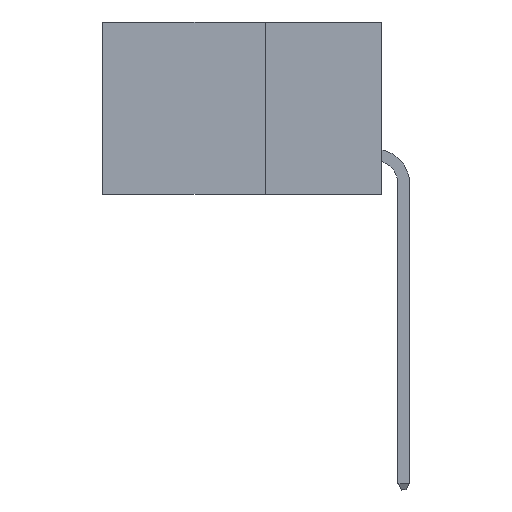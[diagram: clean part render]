
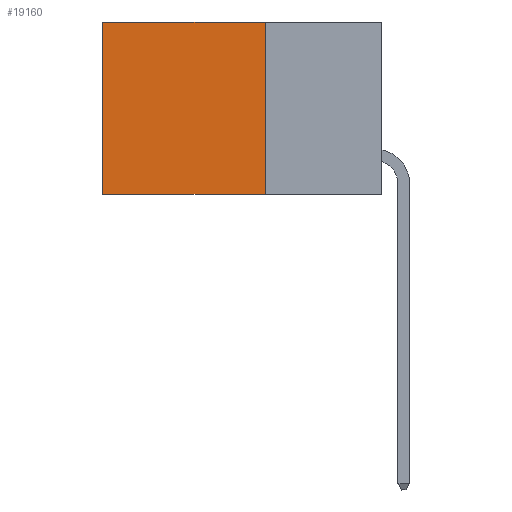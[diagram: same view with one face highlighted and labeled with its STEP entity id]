
A CAD part, left-side view. The second image highlights one B-rep face of the part: STEP entity #19160.
In plain terms, the highlighted planar face has unit normal (-1, 0, 0).
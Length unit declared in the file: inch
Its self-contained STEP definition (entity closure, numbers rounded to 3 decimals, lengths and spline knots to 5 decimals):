
#1195 = DIRECTION ( 'NONE',  ( 0., 0., -1. ) ) ;
#1958 = DIRECTION ( 'NONE',  ( 1., 0., 0. ) ) ;
#2060 = LINE ( 'NONE', #19377, #6332 ) ;
#2730 = ORIENTED_EDGE ( 'NONE', *, *, #21074, .F. ) ;
#3706 = CARTESIAN_POINT ( 'NONE',  ( 0.2875, 0.6, -0.37 ) ) ;
#4814 = VERTEX_POINT ( 'NONE', #15889 ) ;
#6022 = VERTEX_POINT ( 'NONE', #20176 ) ;
#6332 = VECTOR ( 'NONE', #10926, 39.37008 ) ;
#6346 = PLANE ( 'NONE',  #7203 ) ;
#6771 = CARTESIAN_POINT ( 'NONE',  ( 0.2875, 0.25, 0. ) ) ;
#6833 = DIRECTION ( 'NONE',  ( 0., 0., -1. ) ) ;
#6837 = LINE ( 'NONE', #13307, #13934 ) ;
#7063 = CARTESIAN_POINT ( 'NONE',  ( 0.2875, 0.25, -0.37 ) ) ;
#7203 = AXIS2_PLACEMENT_3D ( 'NONE', #6771, #1958, #6833 ) ;
#8243 = VECTOR ( 'NONE', #1195, 39.37008 ) ;
#9307 = ORIENTED_EDGE ( 'NONE', *, *, #21287, .T. ) ;
#10860 = ORIENTED_EDGE ( 'NONE', *, *, #20993, .T. ) ;
#10926 = DIRECTION ( 'NONE',  ( 0., 0., -1. ) ) ;
#11757 = DIRECTION ( 'NONE',  ( 0., 1., 0. ) ) ;
#11871 = FACE_OUTER_BOUND ( 'NONE', #16804, .T. ) ;
#13307 = CARTESIAN_POINT ( 'NONE',  ( 0.2875, 0.25, 0. ) ) ;
#13934 = VECTOR ( 'NONE', #11757, 39.37008 ) ;
#14000 = ORIENTED_EDGE ( 'NONE', *, *, #20195, .F. ) ;
#14814 = CARTESIAN_POINT ( 'NONE',  ( 0.2875, 0.25, 0. ) ) ;
#15468 = VERTEX_POINT ( 'NONE', #3706 ) ;
#15889 = CARTESIAN_POINT ( 'NONE',  ( 0.2875, 0.6, 0. ) ) ;
#16804 = EDGE_LOOP ( 'NONE', ( #9307, #2730, #14000, #10860 ) ) ;
#17175 = CARTESIAN_POINT ( 'NONE',  ( 0.2875, 0.25, -0.37 ) ) ;
#17343 = VECTOR ( 'NONE', #18790, 39.37008 ) ;
#17734 = VERTEX_POINT ( 'NONE', #7063 ) ;
#17892 = LINE ( 'NONE', #17175, #17343 ) ;
#18790 = DIRECTION ( 'NONE',  ( 0., 1., 0. ) ) ;
#18952 = LINE ( 'NONE', #14814, #8243 ) ;
#19160 = ADVANCED_FACE ( 'NONE', ( #11871 ), #6346, .F. ) ;
#19377 = CARTESIAN_POINT ( 'NONE',  ( 0.2875, 0.6, 0. ) ) ;
#20176 = CARTESIAN_POINT ( 'NONE',  ( 0.2875, 0.25, 0. ) ) ;
#20195 = EDGE_CURVE ( 'NONE', #6022, #17734, #18952, .T. ) ;
#20993 = EDGE_CURVE ( 'NONE', #6022, #4814, #6837, .T. ) ;
#21074 = EDGE_CURVE ( 'NONE', #17734, #15468, #17892, .T. ) ;
#21287 = EDGE_CURVE ( 'NONE', #4814, #15468, #2060, .T. ) ;
